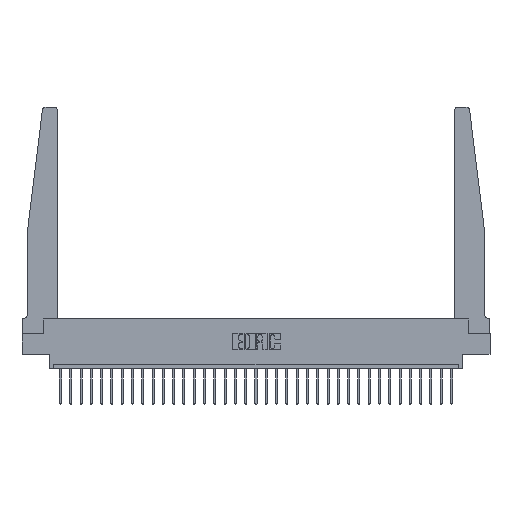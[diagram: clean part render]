
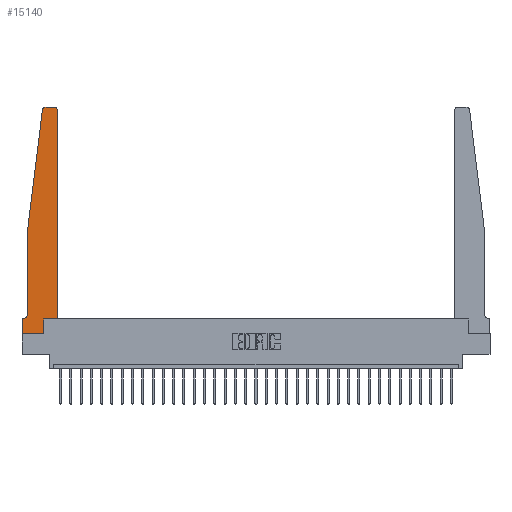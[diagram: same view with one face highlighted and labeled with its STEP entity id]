
A CAD part, top view. The second image highlights one B-rep face of the part: STEP entity #15140.
In plain terms, the highlighted planar face has unit normal (0, 0, 1).
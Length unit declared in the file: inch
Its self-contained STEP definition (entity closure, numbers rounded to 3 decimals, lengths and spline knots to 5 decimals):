
#114 = VECTOR ( 'NONE', #1022, 39.37008 ) ;
#730 = DIRECTION ( 'NONE',  ( -1., 0., 0. ) ) ;
#913 = CARTESIAN_POINT ( 'NONE',  ( 0.065, 1.25, 0.37 ) ) ;
#1003 = DIRECTION ( 'NONE',  ( 0., -1., 0. ) ) ;
#1022 = DIRECTION ( 'NONE',  ( 0., 1., 0. ) ) ;
#1048 = ORIENTED_EDGE ( 'NONE', *, *, #20724, .T. ) ;
#1084 = PLANE ( 'NONE',  #22556 ) ;
#2659 = VECTOR ( 'NONE', #2723, 39.37008 ) ;
#2723 = DIRECTION ( 'NONE',  ( -0.122, -0.992, 0. ) ) ;
#3172 = CARTESIAN_POINT ( 'NONE',  ( 0., 0.1875, 0.37 ) ) ;
#3508 = AXIS2_PLACEMENT_3D ( 'NONE', #19523, #15273, #13127 ) ;
#3650 = DIRECTION ( 'NONE',  ( 0., 0., 1. ) ) ;
#4738 = LINE ( 'NONE', #11687, #7078 ) ;
#4946 = ORIENTED_EDGE ( 'NONE', *, *, #21676, .T. ) ;
#5119 = VERTEX_POINT ( 'NONE', #29695 ) ;
#5588 = DIRECTION ( 'NONE',  ( 1., 0., 0. ) ) ;
#5758 = DIRECTION ( 'NONE',  ( 1., 0., 0. ) ) ;
#6363 = EDGE_CURVE ( 'NONE', #7896, #5119, #14661, .T. ) ;
#6640 = CARTESIAN_POINT ( 'NONE',  ( 0.2605, 0.18, 0.37 ) ) ;
#7078 = VECTOR ( 'NONE', #7582, 39.37008 ) ;
#7582 = DIRECTION ( 'NONE',  ( 1., 0., 0. ) ) ;
#7657 = ORIENTED_EDGE ( 'NONE', *, *, #6363, .T. ) ;
#7896 = VERTEX_POINT ( 'NONE', #8756 ) ;
#8089 = AXIS2_PLACEMENT_3D ( 'NONE', #9834, #3650, #12270 ) ;
#8197 = ORIENTED_EDGE ( 'NONE', *, *, #25840, .T. ) ;
#8469 = EDGE_CURVE ( 'NONE', #22883, #12913, #4738, .T. ) ;
#8756 = CARTESIAN_POINT ( 'NONE',  ( 0.065, 1.25, 0.37 ) ) ;
#9041 = VERTEX_POINT ( 'NONE', #12572 ) ;
#9834 = CARTESIAN_POINT ( 'NONE',  ( 0.27653, 2.72, 0.37 ) ) ;
#9896 = VECTOR ( 'NONE', #5758, 39.37008 ) ;
#9925 = LINE ( 'NONE', #14183, #22748 ) ;
#10101 = DIRECTION ( 'NONE',  ( 0., -1., 0. ) ) ;
#10735 = LINE ( 'NONE', #20017, #27829 ) ;
#11297 = AXIS2_PLACEMENT_3D ( 'NONE', #21176, #16292, #23424 ) ;
#11321 = VECTOR ( 'NONE', #10101, 39.37008 ) ;
#11421 = VERTEX_POINT ( 'NONE', #22405 ) ;
#11439 = CARTESIAN_POINT ( 'NONE',  ( 0.425, 0.18, 0.37 ) ) ;
#11687 = CARTESIAN_POINT ( 'NONE',  ( 0.425, 0.18, 0.37 ) ) ;
#11757 = EDGE_CURVE ( 'NONE', #11421, #22883, #12482, .T. ) ;
#12084 = DIRECTION ( 'NONE',  ( 0., 0., 1. ) ) ;
#12270 = DIRECTION ( 'NONE',  ( 1., 0., 0. ) ) ;
#12482 = LINE ( 'NONE', #26605, #114 ) ;
#12572 = CARTESIAN_POINT ( 'NONE',  ( 0.27653, 2.75, 0.37 ) ) ;
#12683 = EDGE_CURVE ( 'NONE', #12806, #26785, #25978, .T. ) ;
#12806 = VERTEX_POINT ( 'NONE', #25269 ) ;
#12913 = VERTEX_POINT ( 'NONE', #11439 ) ;
#13127 = DIRECTION ( 'NONE',  ( -1., 0., 0. ) ) ;
#13258 = VECTOR ( 'NONE', #15019, 39.37008 ) ;
#13370 = VERTEX_POINT ( 'NONE', #18949 ) ;
#13716 = CIRCLE ( 'NONE', #11297, 0.03 ) ;
#14145 = ORIENTED_EDGE ( 'NONE', *, *, #21436, .T. ) ;
#14183 = CARTESIAN_POINT ( 'NONE',  ( 0.25, 2.75, 0.37 ) ) ;
#14204 = EDGE_CURVE ( 'NONE', #19679, #9041, #9925, .T. ) ;
#14661 = LINE ( 'NONE', #913, #11321 ) ;
#14890 = CIRCLE ( 'NONE', #8089, 0.03 ) ;
#15019 = DIRECTION ( 'NONE',  ( 0., 1., 0. ) ) ;
#15140 = ADVANCED_FACE ( 'NONE', ( #26061 ), #1084, .T. ) ;
#15238 = VERTEX_POINT ( 'NONE', #28499 ) ;
#15273 = DIRECTION ( 'NONE',  ( 0., 0., -1. ) ) ;
#15779 = ORIENTED_EDGE ( 'NONE', *, *, #19407, .T. ) ;
#16292 = DIRECTION ( 'NONE',  ( 0., 0., 1. ) ) ;
#16805 = EDGE_CURVE ( 'NONE', #5119, #24681, #18977, .T. ) ;
#17016 = CARTESIAN_POINT ( 'NONE',  ( 0., 0., 0.37 ) ) ;
#17076 = CARTESIAN_POINT ( 'NONE',  ( 0.065, 1.25, 0.37 ) ) ;
#17421 = CARTESIAN_POINT ( 'NONE',  ( 0.425, 0.18, 0.37 ) ) ;
#17885 = VECTOR ( 'NONE', #1003, 39.37008 ) ;
#18151 = CARTESIAN_POINT ( 'NONE',  ( 0.015, 0.1875, 0.37 ) ) ;
#18949 = CARTESIAN_POINT ( 'NONE',  ( 0.24675, 2.72367, 0.37 ) ) ;
#18977 = CIRCLE ( 'NONE', #3508, 0.05 ) ;
#19016 = EDGE_LOOP ( 'NONE', ( #26545, #8197, #15779, #7657, #24988, #4946, #25963, #25327, #20187, #19378, #14145, #1048 ) ) ;
#19378 = ORIENTED_EDGE ( 'NONE', *, *, #8469, .T. ) ;
#19407 = EDGE_CURVE ( 'NONE', #13370, #7896, #26193, .T. ) ;
#19523 = CARTESIAN_POINT ( 'NONE',  ( 0.015, 0.2375, 0.37 ) ) ;
#19679 = VERTEX_POINT ( 'NONE', #27398 ) ;
#20017 = CARTESIAN_POINT ( 'NONE',  ( 0.065, 0.1875, 0.37 ) ) ;
#20065 = CARTESIAN_POINT ( 'NONE',  ( 0., 0., 0.37 ) ) ;
#20187 = ORIENTED_EDGE ( 'NONE', *, *, #11757, .T. ) ;
#20724 = EDGE_CURVE ( 'NONE', #15238, #19679, #13716, .T. ) ;
#21176 = CARTESIAN_POINT ( 'NONE',  ( 0.395, 2.72, 0.37 ) ) ;
#21436 = EDGE_CURVE ( 'NONE', #12913, #15238, #28672, .T. ) ;
#21462 = EDGE_CURVE ( 'NONE', #26785, #11421, #21720, .T. ) ;
#21676 = EDGE_CURVE ( 'NONE', #24681, #12806, #10735, .T. ) ;
#21720 = LINE ( 'NONE', #26400, #9896 ) ;
#22405 = CARTESIAN_POINT ( 'NONE',  ( 0.2605, 0., 0.37 ) ) ;
#22556 = AXIS2_PLACEMENT_3D ( 'NONE', #3172, #12084, #5588 ) ;
#22748 = VECTOR ( 'NONE', #730, 39.37008 ) ;
#22883 = VERTEX_POINT ( 'NONE', #6640 ) ;
#23424 = DIRECTION ( 'NONE',  ( 1., 0., 0. ) ) ;
#24681 = VERTEX_POINT ( 'NONE', #18151 ) ;
#24988 = ORIENTED_EDGE ( 'NONE', *, *, #16805, .T. ) ;
#25269 = CARTESIAN_POINT ( 'NONE',  ( 0., 0.1875, 0.37 ) ) ;
#25327 = ORIENTED_EDGE ( 'NONE', *, *, #21462, .T. ) ;
#25840 = EDGE_CURVE ( 'NONE', #9041, #13370, #14890, .T. ) ;
#25963 = ORIENTED_EDGE ( 'NONE', *, *, #12683, .T. ) ;
#25978 = LINE ( 'NONE', #17016, #17885 ) ;
#26061 = FACE_OUTER_BOUND ( 'NONE', #19016, .T. ) ;
#26193 = LINE ( 'NONE', #17076, #2659 ) ;
#26400 = CARTESIAN_POINT ( 'NONE',  ( 0., 0., 0.37 ) ) ;
#26545 = ORIENTED_EDGE ( 'NONE', *, *, #14204, .T. ) ;
#26605 = CARTESIAN_POINT ( 'NONE',  ( 0.2605, 0.18, 0.37 ) ) ;
#26785 = VERTEX_POINT ( 'NONE', #20065 ) ;
#27398 = CARTESIAN_POINT ( 'NONE',  ( 0.395, 2.75, 0.37 ) ) ;
#27829 = VECTOR ( 'NONE', #29262, 39.37008 ) ;
#28499 = CARTESIAN_POINT ( 'NONE',  ( 0.425, 2.72, 0.37 ) ) ;
#28672 = LINE ( 'NONE', #17421, #13258 ) ;
#29262 = DIRECTION ( 'NONE',  ( -1., 0., 0. ) ) ;
#29695 = CARTESIAN_POINT ( 'NONE',  ( 0.065, 0.2375, 0.37 ) ) ;
